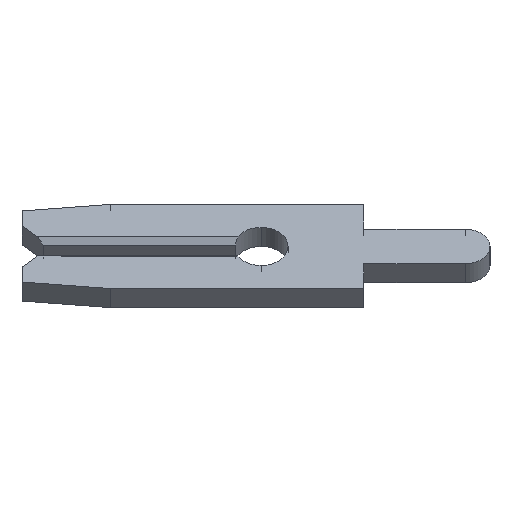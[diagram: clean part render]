
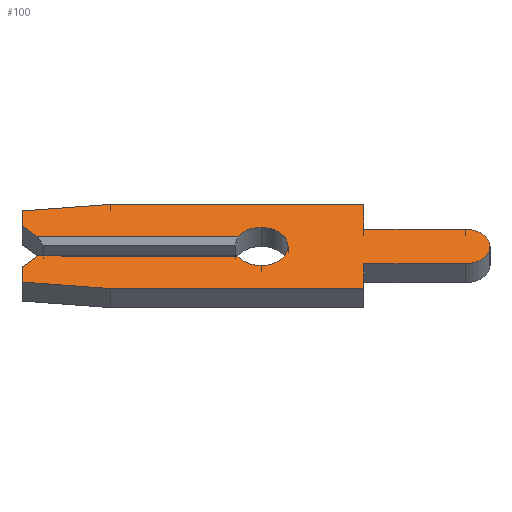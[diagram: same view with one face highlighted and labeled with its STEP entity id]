
A CAD part, left-side view. The second image highlights one B-rep face of the part: STEP entity #100.
In plain terms, the highlighted face is planar.
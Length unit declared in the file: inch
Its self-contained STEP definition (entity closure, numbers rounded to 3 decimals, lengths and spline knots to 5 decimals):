
#1 = VERTEX_POINT ( 'NONE', #1336 ) ;
#5 = VECTOR ( 'NONE', #1258, 39.37008 ) ;
#13 = CARTESIAN_POINT ( 'NONE',  ( -0.013, 0.146, 0.0575 ) ) ;
#33 = ORIENTED_EDGE ( 'NONE', *, *, #1123, .F. ) ;
#62 = VERTEX_POINT ( 'NONE', #210 ) ;
#64 = EDGE_CURVE ( 'NONE', #1, #552, #1166, .T. ) ;
#68 = ORIENTED_EDGE ( 'NONE', *, *, #1286, .F. ) ;
#69 = LINE ( 'NONE', #469, #647 ) ;
#70 = DIRECTION ( 'NONE',  ( 0., -1., 0. ) ) ;
#77 = CARTESIAN_POINT ( 'NONE',  ( -0.013, 0., 0. ) ) ;
#85 = DIRECTION ( 'NONE',  ( 0., 0., -1. ) ) ;
#88 = CARTESIAN_POINT ( 'NONE',  ( -0.013, 0.231, -0.04857 ) ) ;
#90 = VERTEX_POINT ( 'NONE', #998 ) ;
#100 = ADVANCED_FACE ( 'NONE', ( #866 ), #750, .F. ) ;
#112 = LINE ( 'NONE', #300, #616 ) ;
#120 = EDGE_CURVE ( 'NONE', #552, #830, #1285, .T. ) ;
#132 = EDGE_CURVE ( 'NONE', #229, #1351, #741, .T. ) ;
#133 = DIRECTION ( 'NONE',  ( 0., 0., 1. ) ) ;
#148 = VERTEX_POINT ( 'NONE', #340 ) ;
#153 = ORIENTED_EDGE ( 'NONE', *, *, #837, .F. ) ;
#154 = DIRECTION ( 'NONE',  ( 0., 1., 0. ) ) ;
#161 = VERTEX_POINT ( 'NONE', #1012 ) ;
#172 = ORIENTED_EDGE ( 'NONE', *, *, #535, .F. ) ;
#173 = ORIENTED_EDGE ( 'NONE', *, *, #642, .F. ) ;
#181 = VECTOR ( 'NONE', #646, 39.37008 ) ;
#190 = DIRECTION ( 'NONE',  ( 1., 0., 0. ) ) ;
#195 = ORIENTED_EDGE ( 'NONE', *, *, #120, .F. ) ;
#210 = CARTESIAN_POINT ( 'NONE',  ( -0.013, -0.099, -0.0575 ) ) ;
#212 = CARTESIAN_POINT ( 'NONE',  ( -0.013, 0.216, -0.013 ) ) ;
#229 = VERTEX_POINT ( 'NONE', #429 ) ;
#239 = AXIS2_PLACEMENT_3D ( 'NONE', #387, #1292, #371 ) ;
#264 = CARTESIAN_POINT ( 'NONE',  ( -0.013, 0., 0.026 ) ) ;
#273 = EDGE_CURVE ( 'NONE', #62, #628, #385, .T. ) ;
#290 = ORIENTED_EDGE ( 'NONE', *, *, #1049, .T. ) ;
#300 = CARTESIAN_POINT ( 'NONE',  ( -0.013, 0.2105, 0.0075 ) ) ;
#316 = CARTESIAN_POINT ( 'NONE',  ( -0.013, -0.099, 0.0575 ) ) ;
#322 = DIRECTION ( 'NONE',  ( 0., 0., -1. ) ) ;
#340 = CARTESIAN_POINT ( 'NONE',  ( -0.013, 0.02252, 0.013 ) ) ;
#345 = DIRECTION ( 'NONE',  ( 0., 0., -1. ) ) ;
#356 = VERTEX_POINT ( 'NONE', #13 ) ;
#363 = EDGE_CURVE ( 'NONE', #1393, #356, #1366, .T. ) ;
#364 = AXIS2_PLACEMENT_3D ( 'NONE', #648, #1447, #85 ) ;
#368 = CIRCLE ( 'NONE', #239, 0.0235 ) ;
#371 = DIRECTION ( 'NONE',  ( 0., 0., 1. ) ) ;
#385 = LINE ( 'NONE', #1229, #711 ) ;
#387 = CARTESIAN_POINT ( 'NONE',  ( -0.013, -0.1975, 0. ) ) ;
#401 = ORIENTED_EDGE ( 'NONE', *, *, #1211, .F. ) ;
#411 = CARTESIAN_POINT ( 'NONE',  ( -0.013, 0.231, 0.013 ) ) ;
#426 = CARTESIAN_POINT ( 'NONE',  ( -0.013, 0., -0.013 ) ) ;
#429 = CARTESIAN_POINT ( 'NONE',  ( -0.013, 0.231, -0.028 ) ) ;
#434 = EDGE_CURVE ( 'NONE', #706, #1393, #69, .T. ) ;
#439 = LINE ( 'NONE', #512, #815 ) ;
#469 = CARTESIAN_POINT ( 'NONE',  ( -0.013, 0.231, 0.028 ) ) ;
#474 = VECTOR ( 'NONE', #1175, 39.37008 ) ;
#497 = CARTESIAN_POINT ( 'NONE',  ( -0.013, 0.231, -0.04857 ) ) ;
#499 = VERTEX_POINT ( 'NONE', #705 ) ;
#507 = AXIS2_PLACEMENT_3D ( 'NONE', #77, #190, #1101 ) ;
#512 = CARTESIAN_POINT ( 'NONE',  ( -0.013, 0.146, 0.0575 ) ) ;
#535 = EDGE_CURVE ( 'NONE', #830, #148, #772, .T. ) ;
#552 = VERTEX_POINT ( 'NONE', #572 ) ;
#560 = VECTOR ( 'NONE', #633, 39.37008 ) ;
#572 = CARTESIAN_POINT ( 'NONE',  ( -0.013, 0., -0.026 ) ) ;
#590 = ORIENTED_EDGE ( 'NONE', *, *, #273, .F. ) ;
#591 = CARTESIAN_POINT ( 'NONE',  ( -0.013, 0.231, -0.028 ) ) ;
#616 = VECTOR ( 'NONE', #1331, 39.37008 ) ;
#622 = ORIENTED_EDGE ( 'NONE', *, *, #1300, .F. ) ;
#628 = VERTEX_POINT ( 'NONE', #720 ) ;
#629 = LINE ( 'NONE', #714, #938 ) ;
#633 = DIRECTION ( 'NONE',  ( 0., -1., 0. ) ) ;
#635 = VERTEX_POINT ( 'NONE', #1282 ) ;
#642 = EDGE_CURVE ( 'NONE', #1053, #161, #629, .T. ) ;
#646 = DIRECTION ( 'NONE',  ( 0., 0.995, 0.105 ) ) ;
#647 = VECTOR ( 'NONE', #133, 39.37008 ) ;
#648 = CARTESIAN_POINT ( 'NONE',  ( -0.013, 0., 0. ) ) ;
#666 = AXIS2_PLACEMENT_3D ( 'NONE', #682, #780, #792 ) ;
#671 = LINE ( 'NONE', #591, #474 ) ;
#682 = CARTESIAN_POINT ( 'NONE',  ( -0.013, 0., 0. ) ) ;
#690 = LINE ( 'NONE', #1084, #1380 ) ;
#696 = EDGE_LOOP ( 'NONE', ( #290, #172, #195, #831, #1405, #1227, #1096, #622, #590, #1064, #173, #153, #33, #850, #401, #1152, #1042, #68 ) ) ;
#705 = CARTESIAN_POINT ( 'NONE',  ( -0.013, -0.1975, 0.0235 ) ) ;
#706 = VERTEX_POINT ( 'NONE', #952 ) ;
#711 = VECTOR ( 'NONE', #787, 39.37008 ) ;
#714 = CARTESIAN_POINT ( 'NONE',  ( -0.013, -0.099, -0.0235 ) ) ;
#720 = CARTESIAN_POINT ( 'NONE',  ( -0.013, 0.146, -0.0575 ) ) ;
#733 = CARTESIAN_POINT ( 'NONE',  ( -0.013, -0.099, 0.0235 ) ) ;
#741 = LINE ( 'NONE', #893, #1394 ) ;
#750 = PLANE ( 'NONE',  #507 ) ;
#752 = CARTESIAN_POINT ( 'NONE',  ( -0.013, 0.231, 0.04857 ) ) ;
#767 = EDGE_CURVE ( 'NONE', #791, #229, #671, .T. ) ;
#772 = CIRCLE ( 'NONE', #875, 0.026 ) ;
#780 = DIRECTION ( 'NONE',  ( -1., 0., 0. ) ) ;
#787 = DIRECTION ( 'NONE',  ( 0., 1., 0. ) ) ;
#791 = VERTEX_POINT ( 'NONE', #497 ) ;
#792 = DIRECTION ( 'NONE',  ( 0., 0., -1. ) ) ;
#795 = LINE ( 'NONE', #426, #1050 ) ;
#807 = CARTESIAN_POINT ( 'NONE',  ( -0.013, 0.231, 0.04857 ) ) ;
#815 = VECTOR ( 'NONE', #857, 39.37008 ) ;
#830 = VERTEX_POINT ( 'NONE', #264 ) ;
#831 = ORIENTED_EDGE ( 'NONE', *, *, #64, .F. ) ;
#833 = LINE ( 'NONE', #316, #1274 ) ;
#837 = EDGE_CURVE ( 'NONE', #499, #1053, #368, .T. ) ;
#850 = ORIENTED_EDGE ( 'NONE', *, *, #1047, .F. ) ;
#857 = DIRECTION ( 'NONE',  ( 0., -1., 0. ) ) ;
#866 = FACE_OUTER_BOUND ( 'NONE', #696, .T. ) ;
#875 = AXIS2_PLACEMENT_3D ( 'NONE', #1376, #937, #345 ) ;
#879 = LINE ( 'NONE', #411, #1146 ) ;
#893 = CARTESIAN_POINT ( 'NONE',  ( -0.013, 0.2105, -0.0075 ) ) ;
#937 = DIRECTION ( 'NONE',  ( -1., 0., 0. ) ) ;
#938 = VECTOR ( 'NONE', #154, 39.37008 ) ;
#952 = CARTESIAN_POINT ( 'NONE',  ( -0.013, 0.231, 0.028 ) ) ;
#989 = EDGE_CURVE ( 'NONE', #161, #62, #690, .T. ) ;
#998 = CARTESIAN_POINT ( 'NONE',  ( -0.013, 0.216, 0.013 ) ) ;
#1012 = CARTESIAN_POINT ( 'NONE',  ( -0.013, -0.099, -0.0235 ) ) ;
#1042 = ORIENTED_EDGE ( 'NONE', *, *, #434, .F. ) ;
#1047 = EDGE_CURVE ( 'NONE', #1109, #635, #833, .T. ) ;
#1049 = EDGE_CURVE ( 'NONE', #90, #148, #879, .T. ) ;
#1050 = VECTOR ( 'NONE', #1321, 39.37008 ) ;
#1053 = VERTEX_POINT ( 'NONE', #1317 ) ;
#1064 = ORIENTED_EDGE ( 'NONE', *, *, #989, .F. ) ;
#1081 = LINE ( 'NONE', #88, #181 ) ;
#1084 = CARTESIAN_POINT ( 'NONE',  ( -0.013, -0.099, -0.0575 ) ) ;
#1096 = ORIENTED_EDGE ( 'NONE', *, *, #767, .F. ) ;
#1101 = DIRECTION ( 'NONE',  ( 0., 0., -1. ) ) ;
#1109 = VERTEX_POINT ( 'NONE', #1304 ) ;
#1123 = EDGE_CURVE ( 'NONE', #635, #499, #1168, .T. ) ;
#1146 = VECTOR ( 'NONE', #70, 39.37008 ) ;
#1152 = ORIENTED_EDGE ( 'NONE', *, *, #363, .F. ) ;
#1166 = CIRCLE ( 'NONE', #364, 0.026 ) ;
#1168 = LINE ( 'NONE', #733, #560 ) ;
#1175 = DIRECTION ( 'NONE',  ( 0., 0., 1. ) ) ;
#1211 = EDGE_CURVE ( 'NONE', #356, #1109, #439, .T. ) ;
#1226 = DIRECTION ( 'NONE',  ( 0., -0.707, 0.707 ) ) ;
#1227 = ORIENTED_EDGE ( 'NONE', *, *, #132, .F. ) ;
#1229 = CARTESIAN_POINT ( 'NONE',  ( -0.013, 0.146, -0.0575 ) ) ;
#1258 = DIRECTION ( 'NONE',  ( 0., -0.995, 0.105 ) ) ;
#1274 = VECTOR ( 'NONE', #322, 39.37008 ) ;
#1282 = CARTESIAN_POINT ( 'NONE',  ( -0.013, -0.099, 0.0235 ) ) ;
#1285 = CIRCLE ( 'NONE', #666, 0.026 ) ;
#1286 = EDGE_CURVE ( 'NONE', #90, #706, #112, .T. ) ;
#1292 = DIRECTION ( 'NONE',  ( 1., 0., 0. ) ) ;
#1300 = EDGE_CURVE ( 'NONE', #628, #791, #1081, .T. ) ;
#1304 = CARTESIAN_POINT ( 'NONE',  ( -0.013, -0.099, 0.0575 ) ) ;
#1314 = DIRECTION ( 'NONE',  ( 0., 0., -1. ) ) ;
#1317 = CARTESIAN_POINT ( 'NONE',  ( -0.013, -0.1975, -0.0235 ) ) ;
#1321 = DIRECTION ( 'NONE',  ( 0., -1., 0. ) ) ;
#1331 = DIRECTION ( 'NONE',  ( 0., 0.707, 0.707 ) ) ;
#1336 = CARTESIAN_POINT ( 'NONE',  ( -0.013, 0.02252, -0.013 ) ) ;
#1351 = VERTEX_POINT ( 'NONE', #212 ) ;
#1366 = LINE ( 'NONE', #807, #5 ) ;
#1376 = CARTESIAN_POINT ( 'NONE',  ( -0.013, 0., 0. ) ) ;
#1380 = VECTOR ( 'NONE', #1314, 39.37008 ) ;
#1393 = VERTEX_POINT ( 'NONE', #752 ) ;
#1394 = VECTOR ( 'NONE', #1226, 39.37008 ) ;
#1405 = ORIENTED_EDGE ( 'NONE', *, *, #1419, .F. ) ;
#1419 = EDGE_CURVE ( 'NONE', #1351, #1, #795, .T. ) ;
#1447 = DIRECTION ( 'NONE',  ( -1., 0., 0. ) ) ;
